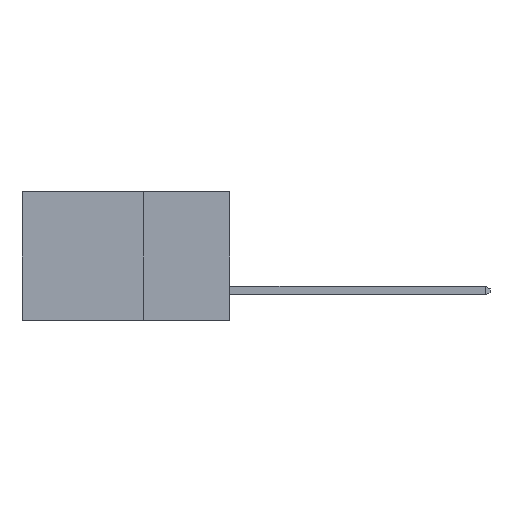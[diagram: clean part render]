
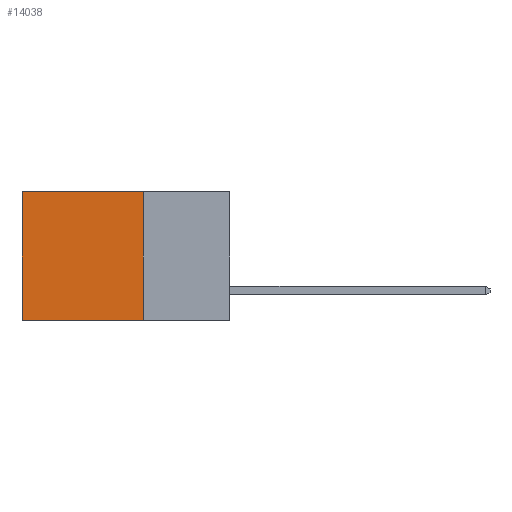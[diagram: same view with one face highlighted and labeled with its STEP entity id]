
A CAD part, left-side view. The second image highlights one B-rep face of the part: STEP entity #14038.
In plain terms, the highlighted planar face has unit normal (-1, 0, 0).
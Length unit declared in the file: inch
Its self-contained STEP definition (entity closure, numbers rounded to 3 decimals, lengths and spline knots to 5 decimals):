
#164 = DIRECTION ( 'NONE',  ( 0., 0., -1. ) ) ;
#392 = CARTESIAN_POINT ( 'NONE',  ( 0.2615, 0.6, 0. ) ) ;
#436 = DIRECTION ( 'NONE',  ( 0., 0., -1. ) ) ;
#919 = AXIS2_PLACEMENT_3D ( 'NONE', #10616, #3470, #164 ) ;
#960 = VECTOR ( 'NONE', #5591, 39.37008 ) ;
#1076 = VECTOR ( 'NONE', #8445, 39.37008 ) ;
#3252 = LINE ( 'NONE', #7244, #1076 ) ;
#3470 = DIRECTION ( 'NONE',  ( 1., 0., 0. ) ) ;
#4747 = FACE_OUTER_BOUND ( 'NONE', #11710, .T. ) ;
#5020 = ORIENTED_EDGE ( 'NONE', *, *, #11402, .F. ) ;
#5033 = CARTESIAN_POINT ( 'NONE',  ( 0.2615, 0.25, -0.37 ) ) ;
#5047 = CARTESIAN_POINT ( 'NONE',  ( 0.2615, 0.6, -0.37 ) ) ;
#5379 = EDGE_CURVE ( 'NONE', #9201, #8474, #3252, .T. ) ;
#5591 = DIRECTION ( 'NONE',  ( 0., 1., 0. ) ) ;
#5922 = DIRECTION ( 'NONE',  ( 0., 1., 0. ) ) ;
#7102 = ORIENTED_EDGE ( 'NONE', *, *, #5379, .T. ) ;
#7244 = CARTESIAN_POINT ( 'NONE',  ( 0.2615, 0.6, -0.37 ) ) ;
#7415 = VECTOR ( 'NONE', #436, 39.37008 ) ;
#7709 = ORIENTED_EDGE ( 'NONE', *, *, #9567, .T. ) ;
#8445 = DIRECTION ( 'NONE',  ( 0., 0., -1. ) ) ;
#8474 = VERTEX_POINT ( 'NONE', #5047 ) ;
#8585 = CARTESIAN_POINT ( 'NONE',  ( 0.2615, 0.25, -0.37 ) ) ;
#9201 = VERTEX_POINT ( 'NONE', #392 ) ;
#9442 = CARTESIAN_POINT ( 'NONE',  ( 0.2615, 0.25, 0. ) ) ;
#9567 = EDGE_CURVE ( 'NONE', #10420, #9201, #10300, .T. ) ;
#9953 = EDGE_CURVE ( 'NONE', #13303, #8474, #14664, .T. ) ;
#10231 = ORIENTED_EDGE ( 'NONE', *, *, #9953, .F. ) ;
#10300 = LINE ( 'NONE', #11559, #960 ) ;
#10420 = VERTEX_POINT ( 'NONE', #9442 ) ;
#10616 = CARTESIAN_POINT ( 'NONE',  ( 0.2615, 0.25, -0.37 ) ) ;
#11402 = EDGE_CURVE ( 'NONE', #10420, #13303, #11624, .T. ) ;
#11559 = CARTESIAN_POINT ( 'NONE',  ( 0.2615, 0.25, 0. ) ) ;
#11624 = LINE ( 'NONE', #5033, #7415 ) ;
#11710 = EDGE_LOOP ( 'NONE', ( #7102, #10231, #5020, #7709 ) ) ;
#11778 = VECTOR ( 'NONE', #5922, 39.37008 ) ;
#12852 = PLANE ( 'NONE',  #919 ) ;
#13303 = VERTEX_POINT ( 'NONE', #14091 ) ;
#14038 = ADVANCED_FACE ( 'NONE', ( #4747 ), #12852, .F. ) ;
#14091 = CARTESIAN_POINT ( 'NONE',  ( 0.2615, 0.25, -0.37 ) ) ;
#14664 = LINE ( 'NONE', #8585, #11778 ) ;
